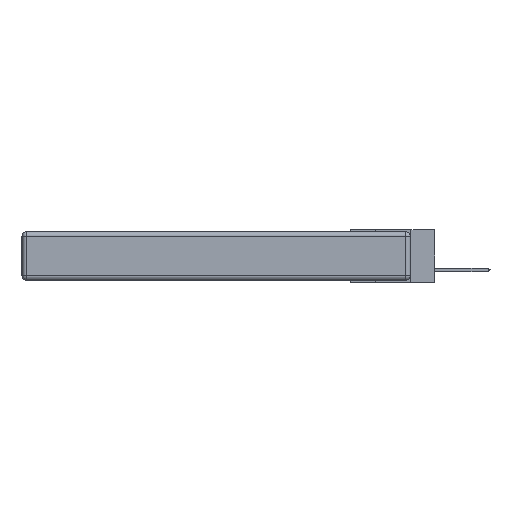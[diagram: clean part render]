
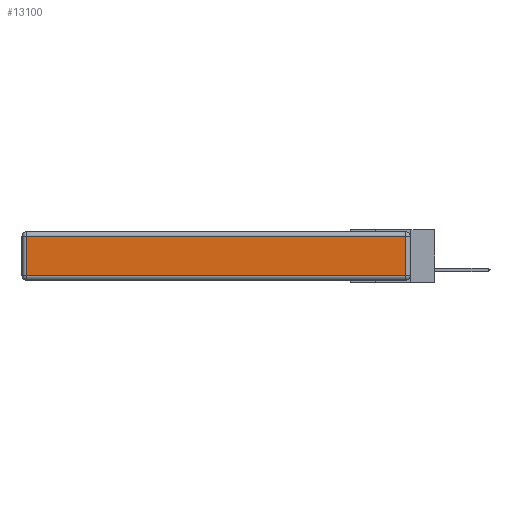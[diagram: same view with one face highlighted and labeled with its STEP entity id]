
A CAD part, left-side view. The second image highlights one B-rep face of the part: STEP entity #13100.
In plain terms, the highlighted planar face has unit normal (-1, 0, 0).
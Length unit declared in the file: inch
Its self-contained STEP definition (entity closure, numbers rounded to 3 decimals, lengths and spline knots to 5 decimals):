
#621 = LINE ( 'NONE', #7948, #18215 ) ;
#657 = CARTESIAN_POINT ( 'NONE',  ( 0., 0.03, -0.343 ) ) ;
#875 = DIRECTION ( 'NONE',  ( -1., 0., 0. ) ) ;
#1027 = DIRECTION ( 'NONE',  ( 0., 0., 1. ) ) ;
#2162 = LINE ( 'NONE', #21825, #8091 ) ;
#2198 = EDGE_CURVE ( 'NONE', #7576, #13406, #12794, .T. ) ;
#2665 = VERTEX_POINT ( 'NONE', #13581 ) ;
#3925 = LINE ( 'NONE', #10461, #16344 ) ;
#4542 = CARTESIAN_POINT ( 'NONE',  ( 0., 0.03, -0.313 ) ) ;
#4664 = CARTESIAN_POINT ( 'NONE',  ( 0., 0., -0.343 ) ) ;
#5700 = DIRECTION ( 'NONE',  ( 0., 1., 0. ) ) ;
#6778 = DIRECTION ( 'NONE',  ( 0., -1., 0. ) ) ;
#7213 = EDGE_LOOP ( 'NONE', ( #16030, #17569, #19693, #18573 ) ) ;
#7576 = VERTEX_POINT ( 'NONE', #4542 ) ;
#7948 = CARTESIAN_POINT ( 'NONE',  ( 0., 2.75, -0.03 ) ) ;
#8091 = VECTOR ( 'NONE', #18465, 39.37008 ) ;
#9183 = DIRECTION ( 'NONE',  ( 0., 0., 1. ) ) ;
#10184 = CARTESIAN_POINT ( 'NONE',  ( 0., 2.72, -0.03 ) ) ;
#10461 = CARTESIAN_POINT ( 'NONE',  ( 0., 0., -0.313 ) ) ;
#10503 = CARTESIAN_POINT ( 'NONE',  ( 0., 0.03, -0.03 ) ) ;
#12180 = VERTEX_POINT ( 'NONE', #10184 ) ;
#12669 = EDGE_CURVE ( 'NONE', #12180, #2665, #2162, .T. ) ;
#12794 = LINE ( 'NONE', #657, #17693 ) ;
#13100 = ADVANCED_FACE ( 'NONE', ( #15912 ), #21796, .T. ) ;
#13406 = VERTEX_POINT ( 'NONE', #10503 ) ;
#13581 = CARTESIAN_POINT ( 'NONE',  ( 0., 2.72, -0.313 ) ) ;
#14117 = AXIS2_PLACEMENT_3D ( 'NONE', #4664, #875, #1027 ) ;
#15912 = FACE_OUTER_BOUND ( 'NONE', #7213, .T. ) ;
#16030 = ORIENTED_EDGE ( 'NONE', *, *, #17217, .T. ) ;
#16344 = VECTOR ( 'NONE', #6778, 39.37008 ) ;
#17217 = EDGE_CURVE ( 'NONE', #2665, #7576, #3925, .T. ) ;
#17569 = ORIENTED_EDGE ( 'NONE', *, *, #2198, .T. ) ;
#17693 = VECTOR ( 'NONE', #9183, 39.37008 ) ;
#18215 = VECTOR ( 'NONE', #5700, 39.37008 ) ;
#18410 = EDGE_CURVE ( 'NONE', #13406, #12180, #621, .T. ) ;
#18465 = DIRECTION ( 'NONE',  ( 0., 0., -1. ) ) ;
#18573 = ORIENTED_EDGE ( 'NONE', *, *, #12669, .T. ) ;
#19693 = ORIENTED_EDGE ( 'NONE', *, *, #18410, .T. ) ;
#21796 = PLANE ( 'NONE',  #14117 ) ;
#21825 = CARTESIAN_POINT ( 'NONE',  ( 0., 2.72, -0.343 ) ) ;
